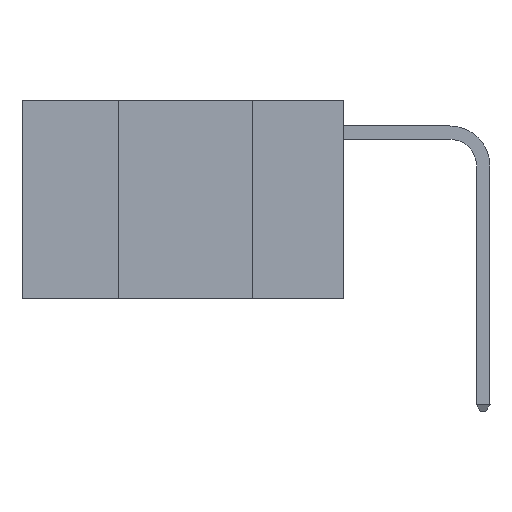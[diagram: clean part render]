
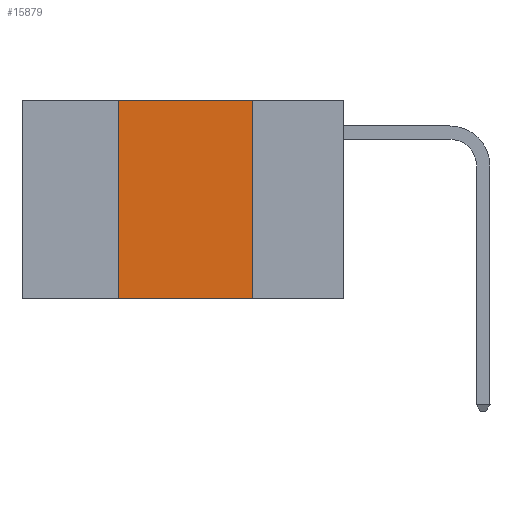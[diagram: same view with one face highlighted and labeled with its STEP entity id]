
A CAD part, left-side view. The second image highlights one B-rep face of the part: STEP entity #15879.
In plain terms, the highlighted planar face has unit normal (-1, 0, 0).
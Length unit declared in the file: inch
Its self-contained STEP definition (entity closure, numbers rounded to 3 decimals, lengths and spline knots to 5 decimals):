
#1056 = DIRECTION ( 'NONE',  ( 0., 0., -1. ) ) ;
#2691 = VECTOR ( 'NONE', #26200, 39.37008 ) ;
#2709 = CARTESIAN_POINT ( 'NONE',  ( 0., 0.42, 0. ) ) ;
#3065 = AXIS2_PLACEMENT_3D ( 'NONE', #22419, #26716, #1056 ) ;
#3334 = CARTESIAN_POINT ( 'NONE',  ( 0., 0.42, 0. ) ) ;
#4078 = VECTOR ( 'NONE', #6385, 39.37008 ) ;
#5498 = DIRECTION ( 'NONE',  ( 0., -1., 0. ) ) ;
#6385 = DIRECTION ( 'NONE',  ( 0., 0., -1. ) ) ;
#6642 = CARTESIAN_POINT ( 'NONE',  ( 0., 0.17, -0.37 ) ) ;
#7505 = CARTESIAN_POINT ( 'NONE',  ( 0., 0.6, 0. ) ) ;
#8053 = EDGE_CURVE ( 'NONE', #12021, #21766, #22904, .T. ) ;
#8641 = CARTESIAN_POINT ( 'NONE',  ( 0., 0.42, -0.37 ) ) ;
#8752 = ORIENTED_EDGE ( 'NONE', *, *, #10927, .F. ) ;
#9230 = ORIENTED_EDGE ( 'NONE', *, *, #8053, .F. ) ;
#9554 = VECTOR ( 'NONE', #5498, 39.37008 ) ;
#9728 = PLANE ( 'NONE',  #3065 ) ;
#9768 = EDGE_CURVE ( 'NONE', #22867, #12021, #20720, .T. ) ;
#10806 = LINE ( 'NONE', #15245, #4078 ) ;
#10927 = EDGE_CURVE ( 'NONE', #21766, #17183, #10806, .T. ) ;
#12021 = VERTEX_POINT ( 'NONE', #2709 ) ;
#15245 = CARTESIAN_POINT ( 'NONE',  ( 0., 0.17, 0. ) ) ;
#15502 = CARTESIAN_POINT ( 'NONE',  ( 0., 0.17, 0. ) ) ;
#15879 = ADVANCED_FACE ( 'NONE', ( #20124 ), #9728, .F. ) ;
#17183 = VERTEX_POINT ( 'NONE', #6642 ) ;
#17810 = DIRECTION ( 'NONE',  ( 0., -1., 0. ) ) ;
#19931 = CARTESIAN_POINT ( 'NONE',  ( 0., 0.6, -0.37 ) ) ;
#20124 = FACE_OUTER_BOUND ( 'NONE', #22271, .T. ) ;
#20720 = LINE ( 'NONE', #3334, #2691 ) ;
#20820 = ORIENTED_EDGE ( 'NONE', *, *, #9768, .F. ) ;
#21766 = VERTEX_POINT ( 'NONE', #15502 ) ;
#21962 = VECTOR ( 'NONE', #17810, 39.37008 ) ;
#22271 = EDGE_LOOP ( 'NONE', ( #8752, #9230, #20820, #27530 ) ) ;
#22419 = CARTESIAN_POINT ( 'NONE',  ( 0., 0.6, 0. ) ) ;
#22867 = VERTEX_POINT ( 'NONE', #8641 ) ;
#22904 = LINE ( 'NONE', #7505, #9554 ) ;
#23883 = EDGE_CURVE ( 'NONE', #22867, #17183, #24677, .T. ) ;
#24677 = LINE ( 'NONE', #19931, #21962 ) ;
#26200 = DIRECTION ( 'NONE',  ( 0., 0., 1. ) ) ;
#26716 = DIRECTION ( 'NONE',  ( 1., 0., 0. ) ) ;
#27530 = ORIENTED_EDGE ( 'NONE', *, *, #23883, .T. ) ;
